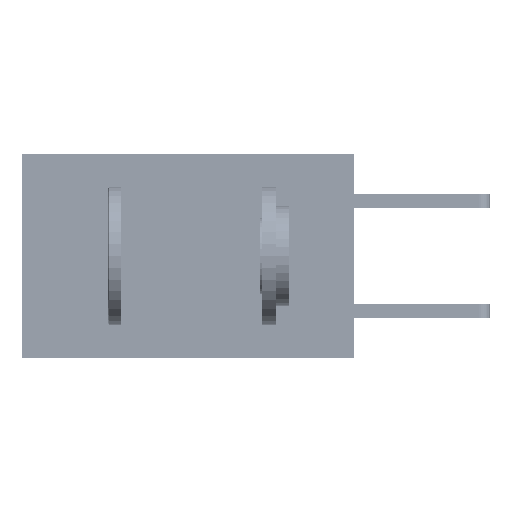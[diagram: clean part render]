
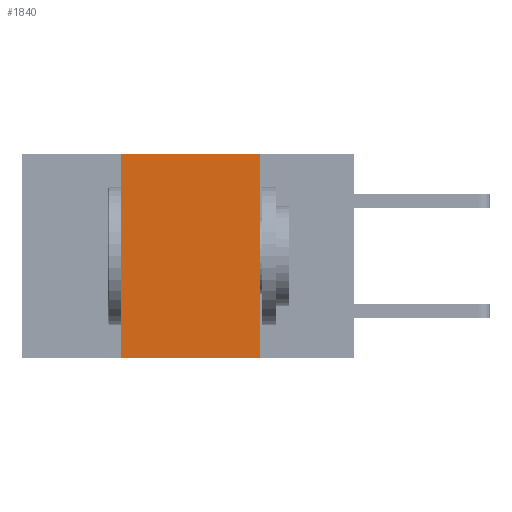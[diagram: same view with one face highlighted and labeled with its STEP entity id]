
A CAD part, left-side view. The second image highlights one B-rep face of the part: STEP entity #1840.
In plain terms, the highlighted planar face has unit normal (-1, 0, 0).
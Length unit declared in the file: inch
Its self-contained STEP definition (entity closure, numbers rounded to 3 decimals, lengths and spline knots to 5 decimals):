
#1217 = CARTESIAN_POINT ( 'NONE',  ( 0., 0.17, -0.37 ) ) ;
#1840 = ADVANCED_FACE ( 'NONE', ( #5098 ), #47862, .F. ) ;
#3246 = AXIS2_PLACEMENT_3D ( 'NONE', #44557, #22084, #18616 ) ;
#4855 = CARTESIAN_POINT ( 'NONE',  ( 0., 0.6, -0.37 ) ) ;
#5057 = EDGE_CURVE ( 'NONE', #47586, #40272, #29134, .T. ) ;
#5098 = FACE_OUTER_BOUND ( 'NONE', #37857, .T. ) ;
#5735 = ORIENTED_EDGE ( 'NONE', *, *, #10172, .T. ) ;
#7743 = DIRECTION ( 'NONE',  ( 0., 0., -1. ) ) ;
#8076 = VERTEX_POINT ( 'NONE', #34703 ) ;
#8301 = CARTESIAN_POINT ( 'NONE',  ( 0., 0.6, 0. ) ) ;
#9255 = VECTOR ( 'NONE', #7743, 39.37008 ) ;
#9304 = VECTOR ( 'NONE', #14488, 39.37008 ) ;
#10172 = EDGE_CURVE ( 'NONE', #8076, #40272, #48184, .T. ) ;
#11161 = VERTEX_POINT ( 'NONE', #41017 ) ;
#11768 = CARTESIAN_POINT ( 'NONE',  ( 0., 0.17, 0. ) ) ;
#12722 = ORIENTED_EDGE ( 'NONE', *, *, #37250, .F. ) ;
#14010 = CARTESIAN_POINT ( 'NONE',  ( 0., 0.42, 0. ) ) ;
#14488 = DIRECTION ( 'NONE',  ( 0., 0., 1. ) ) ;
#14520 = LINE ( 'NONE', #14010, #9304 ) ;
#15021 = ORIENTED_EDGE ( 'NONE', *, *, #5057, .F. ) ;
#15637 = DIRECTION ( 'NONE',  ( 0., -1., 0. ) ) ;
#18616 = DIRECTION ( 'NONE',  ( 0., 0., -1. ) ) ;
#20062 = DIRECTION ( 'NONE',  ( 0., -1., 0. ) ) ;
#22084 = DIRECTION ( 'NONE',  ( 1., 0., 0. ) ) ;
#25707 = EDGE_CURVE ( 'NONE', #11161, #47586, #33349, .T. ) ;
#29134 = LINE ( 'NONE', #45119, #9255 ) ;
#33349 = LINE ( 'NONE', #8301, #46881 ) ;
#34703 = CARTESIAN_POINT ( 'NONE',  ( 0., 0.42, -0.37 ) ) ;
#36706 = ORIENTED_EDGE ( 'NONE', *, *, #25707, .F. ) ;
#37250 = EDGE_CURVE ( 'NONE', #8076, #11161, #14520, .T. ) ;
#37857 = EDGE_LOOP ( 'NONE', ( #15021, #36706, #12722, #5735 ) ) ;
#40272 = VERTEX_POINT ( 'NONE', #1217 ) ;
#41017 = CARTESIAN_POINT ( 'NONE',  ( 0., 0.42, 0. ) ) ;
#44557 = CARTESIAN_POINT ( 'NONE',  ( 0., 0.6, 0. ) ) ;
#45119 = CARTESIAN_POINT ( 'NONE',  ( 0., 0.17, 0. ) ) ;
#46881 = VECTOR ( 'NONE', #15637, 39.37008 ) ;
#47010 = VECTOR ( 'NONE', #20062, 39.37008 ) ;
#47586 = VERTEX_POINT ( 'NONE', #11768 ) ;
#47862 = PLANE ( 'NONE',  #3246 ) ;
#48184 = LINE ( 'NONE', #4855, #47010 ) ;
